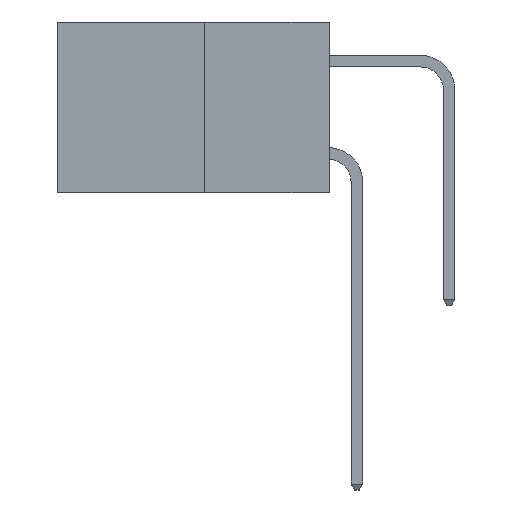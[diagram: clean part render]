
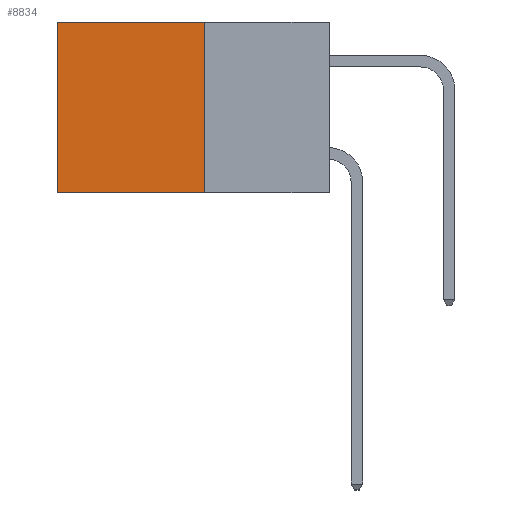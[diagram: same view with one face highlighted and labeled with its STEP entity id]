
A CAD part, left-side view. The second image highlights one B-rep face of the part: STEP entity #8834.
In plain terms, the highlighted planar face has unit normal (-1, 0, 0).
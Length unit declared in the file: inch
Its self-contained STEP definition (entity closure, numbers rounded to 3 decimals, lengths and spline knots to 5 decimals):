
#793 = DIRECTION ( 'NONE',  ( 0., 0., -1. ) ) ;
#808 = ORIENTED_EDGE ( 'NONE', *, *, #902, .T. ) ;
#902 = EDGE_CURVE ( 'NONE', #5095, #17527, #15215, .T. ) ;
#1937 = CARTESIAN_POINT ( 'NONE',  ( 0.277, 0.27, 0. ) ) ;
#2753 = DIRECTION ( 'NONE',  ( 0., 0., -1. ) ) ;
#3208 = ORIENTED_EDGE ( 'NONE', *, *, #20113, .F. ) ;
#3839 = LINE ( 'NONE', #6350, #21889 ) ;
#3930 = ORIENTED_EDGE ( 'NONE', *, *, #15907, .T. ) ;
#4491 = AXIS2_PLACEMENT_3D ( 'NONE', #20039, #11317, #793 ) ;
#5095 = VERTEX_POINT ( 'NONE', #8601 ) ;
#5488 = LINE ( 'NONE', #20115, #14802 ) ;
#5716 = ORIENTED_EDGE ( 'NONE', *, *, #7534, .F. ) ;
#6142 = VECTOR ( 'NONE', #6446, 39.37008 ) ;
#6350 = CARTESIAN_POINT ( 'NONE',  ( 0.277, 0.27, -0.37 ) ) ;
#6446 = DIRECTION ( 'NONE',  ( 0., 1., 0. ) ) ;
#6708 = LINE ( 'NONE', #15212, #6142 ) ;
#7534 = EDGE_CURVE ( 'NONE', #9279, #14952, #3839, .T. ) ;
#8601 = CARTESIAN_POINT ( 'NONE',  ( 0.277, 0.59, 0. ) ) ;
#8834 = ADVANCED_FACE ( 'NONE', ( #19144 ), #9574, .F. ) ;
#8966 = CARTESIAN_POINT ( 'NONE',  ( 0.277, 0.27, -0.37 ) ) ;
#9279 = VERTEX_POINT ( 'NONE', #1937 ) ;
#9574 = PLANE ( 'NONE',  #4491 ) ;
#11317 = DIRECTION ( 'NONE',  ( 1., 0., 0. ) ) ;
#11326 = DIRECTION ( 'NONE',  ( 0., 1., 0. ) ) ;
#13193 = CARTESIAN_POINT ( 'NONE',  ( 0.277, 0.59, -0.37 ) ) ;
#14802 = VECTOR ( 'NONE', #11326, 39.37008 ) ;
#14952 = VERTEX_POINT ( 'NONE', #8966 ) ;
#15212 = CARTESIAN_POINT ( 'NONE',  ( 0.277, 0.27, 0. ) ) ;
#15215 = LINE ( 'NONE', #13193, #19304 ) ;
#15907 = EDGE_CURVE ( 'NONE', #9279, #5095, #6708, .T. ) ;
#17527 = VERTEX_POINT ( 'NONE', #18459 ) ;
#18459 = CARTESIAN_POINT ( 'NONE',  ( 0.277, 0.59, -0.37 ) ) ;
#18462 = EDGE_LOOP ( 'NONE', ( #808, #3208, #5716, #3930 ) ) ;
#19144 = FACE_OUTER_BOUND ( 'NONE', #18462, .T. ) ;
#19304 = VECTOR ( 'NONE', #2753, 39.37008 ) ;
#20039 = CARTESIAN_POINT ( 'NONE',  ( 0.277, 0.27, -0.37 ) ) ;
#20113 = EDGE_CURVE ( 'NONE', #14952, #17527, #5488, .T. ) ;
#20115 = CARTESIAN_POINT ( 'NONE',  ( 0.277, 0.27, -0.37 ) ) ;
#20384 = DIRECTION ( 'NONE',  ( 0., 0., -1. ) ) ;
#21889 = VECTOR ( 'NONE', #20384, 39.37008 ) ;
